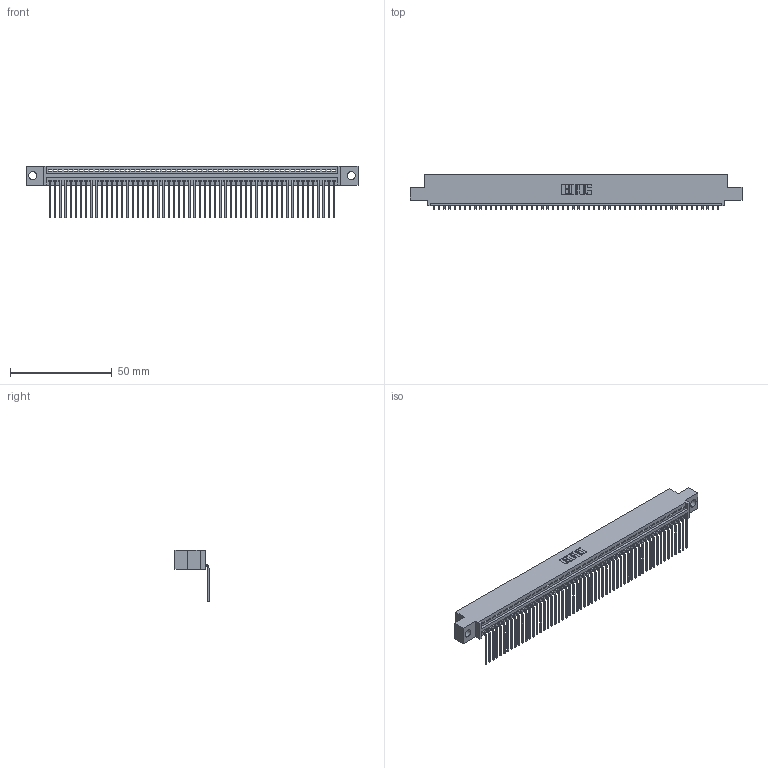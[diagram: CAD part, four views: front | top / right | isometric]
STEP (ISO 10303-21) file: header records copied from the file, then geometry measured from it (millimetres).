
FILE_DESCRIPTION (( 'STEP AP203' ), '1' );
FILE_NAME ('345-056-559-404.STEP', '2018-09-25T20:57:10', ( '' ), ( '' ), 'SwSTEP 2.0', 'SolidWorks 2016', '' );
FILE_SCHEMA (( 'CONFIG_CONTROL_DESIGN' ));
Length unit declared in the file: inch
Products named in the file (3): 345-056-559-404; 345 Part_0.110 Offset - 0.156 Dia-TH; 345-292-001_558 559 Tail - 1
Assembly tree (57 placements, depth 2):
  345-056-559-404
    345 Part_0.110 Offset - 0.156 Dia-TH
    345-292-001_558 559 Tail - 1  x56
Bounding box: 163.45 x 16.75 x 25.53 mm (x, y, z)
Volume: 15664.6 mm3; surface area: 21994.1 mm2
Topology: 57 solids, 57 shells, 3490 faces, 10545 edges, 6954 vertices
Faces by surface type: plane 2436, cylinder 1054
Entity records: 40481 total; most frequent: CARTESIAN_POINT 7020, ORIENTED_EDGE 7010, DIRECTION 6109, EDGE_CURVE 3505, LINE 3149, VECTOR 3149, VERTEX_POINT 2334, AXIS2_PLACEMENT_3D 1480
